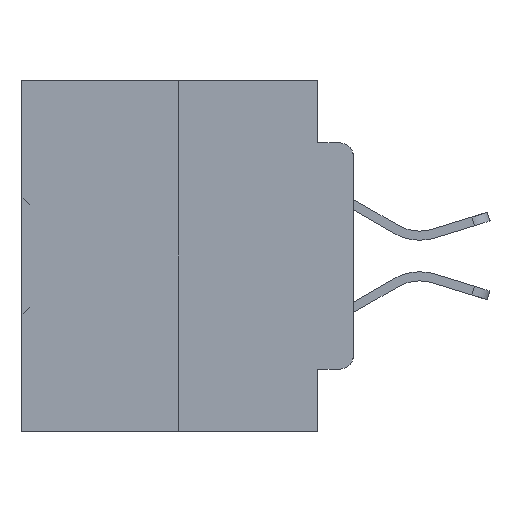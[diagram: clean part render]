
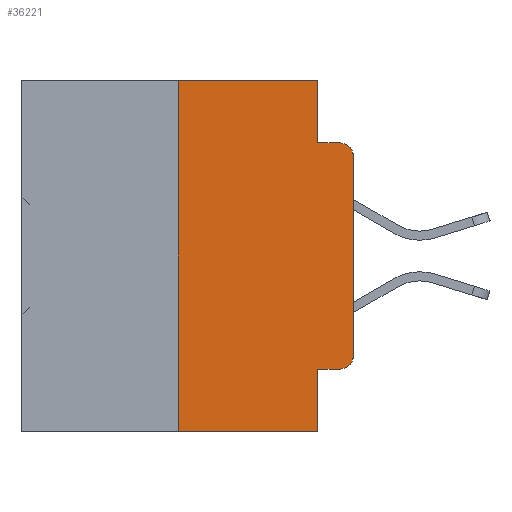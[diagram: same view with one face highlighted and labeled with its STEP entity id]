
A CAD part, left-side view. The second image highlights one B-rep face of the part: STEP entity #36221.
In plain terms, the highlighted planar face has unit normal (-1, 0, 0).
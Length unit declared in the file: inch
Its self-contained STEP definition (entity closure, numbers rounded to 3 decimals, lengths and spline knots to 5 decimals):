
#101 = CARTESIAN_POINT ( 'NONE',  ( 0., 0.473, 0. ) ) ;
#157 = VERTEX_POINT ( 'NONE', #7137 ) ;
#950 = LINE ( 'NONE', #25747, #12097 ) ;
#1458 = ORIENTED_EDGE ( 'NONE', *, *, #14627, .T. ) ;
#2351 = LINE ( 'NONE', #7667, #16426 ) ;
#2543 = EDGE_CURVE ( 'NONE', #11539, #15701, #37060, .T. ) ;
#2887 = DIRECTION ( 'NONE',  ( 0., -1., 0. ) ) ;
#3194 = VECTOR ( 'NONE', #8007, 39.37008 ) ;
#4730 = VERTEX_POINT ( 'NONE', #27603 ) ;
#5190 = VERTEX_POINT ( 'NONE', #33822 ) ;
#5476 = VECTOR ( 'NONE', #2887, 39.37008 ) ;
#6606 = CARTESIAN_POINT ( 'NONE',  ( 0., 0.02, -0.0885 ) ) ;
#6833 = ORIENTED_EDGE ( 'NONE', *, *, #31913, .T. ) ;
#7137 = CARTESIAN_POINT ( 'NONE',  ( 0., 0.25, 0. ) ) ;
#7667 = CARTESIAN_POINT ( 'NONE',  ( 0., 0.25, 0. ) ) ;
#8007 = DIRECTION ( 'NONE',  ( 0., 0., -1. ) ) ;
#8568 = CARTESIAN_POINT ( 'NONE',  ( 0., 0.051, 0. ) ) ;
#10299 = ORIENTED_EDGE ( 'NONE', *, *, #29699, .T. ) ;
#10491 = VECTOR ( 'NONE', #14851, 39.37008 ) ;
#10639 = DIRECTION ( 'NONE',  ( -1., 0., 0. ) ) ;
#11436 = VERTEX_POINT ( 'NONE', #31802 ) ;
#11533 = ORIENTED_EDGE ( 'NONE', *, *, #30752, .T. ) ;
#11539 = VERTEX_POINT ( 'NONE', #14257 ) ;
#12097 = VECTOR ( 'NONE', #38177, 39.37008 ) ;
#12153 = VECTOR ( 'NONE', #15475, 39.37008 ) ;
#13757 = ORIENTED_EDGE ( 'NONE', *, *, #32394, .T. ) ;
#14257 = CARTESIAN_POINT ( 'NONE',  ( 0., 0.051, -0.4115 ) ) ;
#14627 = EDGE_CURVE ( 'NONE', #4730, #23269, #33739, .T. ) ;
#14788 = EDGE_CURVE ( 'NONE', #35866, #23820, #33235, .T. ) ;
#14851 = DIRECTION ( 'NONE',  ( 0., 0., -1. ) ) ;
#15087 = DIRECTION ( 'NONE',  ( -1., 0., 0. ) ) ;
#15409 = CIRCLE ( 'NONE', #26508, 0.02 ) ;
#15475 = DIRECTION ( 'NONE',  ( 0., -1., 0. ) ) ;
#15701 = VERTEX_POINT ( 'NONE', #39243 ) ;
#15716 = EDGE_CURVE ( 'NONE', #23820, #36469, #21286, .T. ) ;
#15817 = AXIS2_PLACEMENT_3D ( 'NONE', #101, #31029, #18373 ) ;
#16426 = VECTOR ( 'NONE', #20034, 39.37008 ) ;
#16496 = ORIENTED_EDGE ( 'NONE', *, *, #2543, .F. ) ;
#16863 = ORIENTED_EDGE ( 'NONE', *, *, #27106, .F. ) ;
#17555 = EDGE_LOOP ( 'NONE', ( #11533, #6833, #37770, #39611, #16863, #19213, #13757, #16496, #10299, #1458 ) ) ;
#17964 = FACE_OUTER_BOUND ( 'NONE', #17555, .T. ) ;
#18313 = LINE ( 'NONE', #25248, #12153 ) ;
#18373 = DIRECTION ( 'NONE',  ( 0., 0., -1. ) ) ;
#18875 = LINE ( 'NONE', #39889, #23898 ) ;
#18923 = CARTESIAN_POINT ( 'NONE',  ( 0., 0.02, -0.1085 ) ) ;
#19213 = ORIENTED_EDGE ( 'NONE', *, *, #19535, .F. ) ;
#19535 = EDGE_CURVE ( 'NONE', #11436, #157, #2351, .T. ) ;
#20034 = DIRECTION ( 'NONE',  ( 0., 0., 1. ) ) ;
#21171 = LINE ( 'NONE', #36670, #5476 ) ;
#21286 = LINE ( 'NONE', #31290, #34457 ) ;
#21364 = AXIS2_PLACEMENT_3D ( 'NONE', #25900, #10639, #35289 ) ;
#23269 = VERTEX_POINT ( 'NONE', #24292 ) ;
#23820 = VERTEX_POINT ( 'NONE', #39729 ) ;
#23898 = VECTOR ( 'NONE', #24201, 39.37008 ) ;
#24052 = CARTESIAN_POINT ( 'NONE',  ( 0., 0.051, 0. ) ) ;
#24201 = DIRECTION ( 'NONE',  ( 0., -1., 0. ) ) ;
#24292 = CARTESIAN_POINT ( 'NONE',  ( 0., 0., -0.3915 ) ) ;
#25248 = CARTESIAN_POINT ( 'NONE',  ( 0., 0.051, -0.4115 ) ) ;
#25747 = CARTESIAN_POINT ( 'NONE',  ( 0., 0., 0. ) ) ;
#25900 = CARTESIAN_POINT ( 'NONE',  ( 0., 0.02, -0.3915 ) ) ;
#26508 = AXIS2_PLACEMENT_3D ( 'NONE', #18923, #15087, #39940 ) ;
#27106 = EDGE_CURVE ( 'NONE', #157, #35866, #21171, .T. ) ;
#27603 = CARTESIAN_POINT ( 'NONE',  ( 0., 0.02, -0.4115 ) ) ;
#28233 = CARTESIAN_POINT ( 'NONE',  ( 0., 0.051, 0. ) ) ;
#29699 = EDGE_CURVE ( 'NONE', #11539, #4730, #18313, .T. ) ;
#30232 = PLANE ( 'NONE',  #15817 ) ;
#30752 = EDGE_CURVE ( 'NONE', #23269, #5190, #950, .T. ) ;
#31029 = DIRECTION ( 'NONE',  ( 1., 0., 0. ) ) ;
#31290 = CARTESIAN_POINT ( 'NONE',  ( 0., 0.051, -0.0885 ) ) ;
#31802 = CARTESIAN_POINT ( 'NONE',  ( 0., 0.25, -0.5 ) ) ;
#31913 = EDGE_CURVE ( 'NONE', #5190, #36469, #15409, .T. ) ;
#32394 = EDGE_CURVE ( 'NONE', #11436, #15701, #18875, .T. ) ;
#33235 = LINE ( 'NONE', #24052, #3194 ) ;
#33735 = DIRECTION ( 'NONE',  ( 0., -1., 0. ) ) ;
#33739 = CIRCLE ( 'NONE', #21364, 0.02 ) ;
#33822 = CARTESIAN_POINT ( 'NONE',  ( 0., 0., -0.1085 ) ) ;
#34457 = VECTOR ( 'NONE', #33735, 39.37008 ) ;
#35289 = DIRECTION ( 'NONE',  ( 0., 0., -1. ) ) ;
#35866 = VERTEX_POINT ( 'NONE', #28233 ) ;
#36221 = ADVANCED_FACE ( 'NONE', ( #17964 ), #30232, .F. ) ;
#36469 = VERTEX_POINT ( 'NONE', #6606 ) ;
#36670 = CARTESIAN_POINT ( 'NONE',  ( 0., 0.473, 0. ) ) ;
#37060 = LINE ( 'NONE', #8568, #10491 ) ;
#37770 = ORIENTED_EDGE ( 'NONE', *, *, #15716, .F. ) ;
#38177 = DIRECTION ( 'NONE',  ( 0., 0., 1. ) ) ;
#39243 = CARTESIAN_POINT ( 'NONE',  ( 0., 0.051, -0.5 ) ) ;
#39611 = ORIENTED_EDGE ( 'NONE', *, *, #14788, .F. ) ;
#39729 = CARTESIAN_POINT ( 'NONE',  ( 0., 0.051, -0.0885 ) ) ;
#39889 = CARTESIAN_POINT ( 'NONE',  ( 0., 0.473, -0.5 ) ) ;
#39940 = DIRECTION ( 'NONE',  ( 0., 0., -1. ) ) ;
